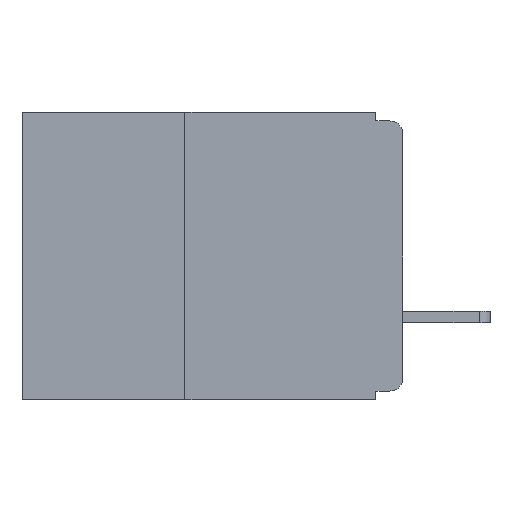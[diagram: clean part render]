
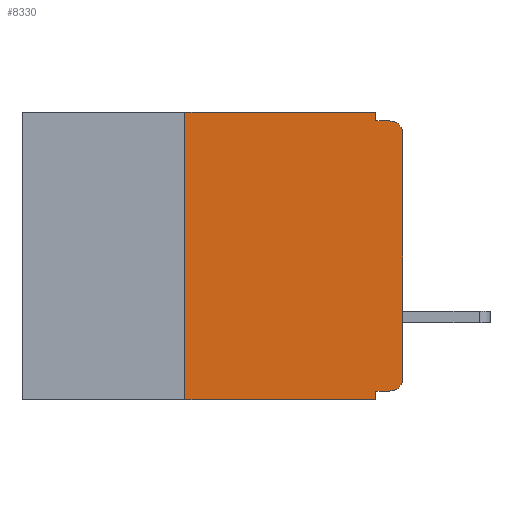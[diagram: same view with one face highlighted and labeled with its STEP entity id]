
A CAD part, left-side view. The second image highlights one B-rep face of the part: STEP entity #8330.
In plain terms, the highlighted planar face has unit normal (-1, 0, 0).
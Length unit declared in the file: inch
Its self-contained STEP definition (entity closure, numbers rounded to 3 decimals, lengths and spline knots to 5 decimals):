
#650 = LINE ( 'NONE', #17248, #4977 ) ;
#675 = ORIENTED_EDGE ( 'NONE', *, *, #1697, .T. ) ;
#850 = EDGE_CURVE ( 'NONE', #20272, #13504, #3624, .T. ) ;
#1159 = VERTEX_POINT ( 'NONE', #6246 ) ;
#1633 = AXIS2_PLACEMENT_3D ( 'NONE', #23522, #14543, #3384 ) ;
#1697 = EDGE_CURVE ( 'NONE', #17178, #10388, #9512, .T. ) ;
#1783 = LINE ( 'NONE', #21911, #15415 ) ;
#2965 = ORIENTED_EDGE ( 'NONE', *, *, #850, .F. ) ;
#3384 = DIRECTION ( 'NONE',  ( 0., 0., -1. ) ) ;
#3624 = LINE ( 'NONE', #14983, #22013 ) ;
#3762 = VERTEX_POINT ( 'NONE', #18606 ) ;
#4073 = LINE ( 'NONE', #21088, #13419 ) ;
#4673 = EDGE_CURVE ( 'NONE', #13071, #1159, #1783, .T. ) ;
#4823 = VECTOR ( 'NONE', #6919, 39.37008 ) ;
#4966 = ORIENTED_EDGE ( 'NONE', *, *, #10461, .T. ) ;
#4977 = VECTOR ( 'NONE', #9965, 39.37008 ) ;
#6220 = VECTOR ( 'NONE', #15174, 39.37008 ) ;
#6246 = CARTESIAN_POINT ( 'NONE',  ( 0., 0.25, 0. ) ) ;
#6919 = DIRECTION ( 'NONE',  ( 0., 1., 0. ) ) ;
#7081 = LINE ( 'NONE', #10183, #16347 ) ;
#7742 = FACE_OUTER_BOUND ( 'NONE', #14845, .T. ) ;
#7944 = CIRCLE ( 'NONE', #21396, 0.015 ) ;
#8330 = ADVANCED_FACE ( 'NONE', ( #7742 ), #16301, .F. ) ;
#9512 = CIRCLE ( 'NONE', #16592, 0.015 ) ;
#9738 = CARTESIAN_POINT ( 'NONE',  ( 0., 0.015, -0.025 ) ) ;
#9762 = CARTESIAN_POINT ( 'NONE',  ( 0., 0.25, -0.33 ) ) ;
#9819 = LINE ( 'NONE', #12503, #4823 ) ;
#9965 = DIRECTION ( 'NONE',  ( 0., -1., 0. ) ) ;
#10183 = CARTESIAN_POINT ( 'NONE',  ( 0., 0., -0.01 ) ) ;
#10388 = VERTEX_POINT ( 'NONE', #15047 ) ;
#10461 = EDGE_CURVE ( 'NONE', #3762, #15652, #7944, .T. ) ;
#11070 = CARTESIAN_POINT ( 'NONE',  ( 0., 0.031, 0. ) ) ;
#11258 = EDGE_CURVE ( 'NONE', #19746, #11695, #4073, .T. ) ;
#11275 = CARTESIAN_POINT ( 'NONE',  ( 0., 0.437, 0. ) ) ;
#11535 = CARTESIAN_POINT ( 'NONE',  ( 0., 0.015, -0.32 ) ) ;
#11639 = DIRECTION ( 'NONE',  ( 0., 0., -1. ) ) ;
#11695 = VERTEX_POINT ( 'NONE', #14999 ) ;
#12277 = CARTESIAN_POINT ( 'NONE',  ( 0., 0.015, -0.01 ) ) ;
#12503 = CARTESIAN_POINT ( 'NONE',  ( 0., 0., -0.32 ) ) ;
#12838 = EDGE_CURVE ( 'NONE', #1159, #19746, #16745, .T. ) ;
#12869 = ORIENTED_EDGE ( 'NONE', *, *, #11258, .F. ) ;
#13071 = VERTEX_POINT ( 'NONE', #9762 ) ;
#13159 = ORIENTED_EDGE ( 'NONE', *, *, #17260, .T. ) ;
#13350 = CARTESIAN_POINT ( 'NONE',  ( 0., 0., 0. ) ) ;
#13419 = VECTOR ( 'NONE', #22865, 39.37008 ) ;
#13504 = VERTEX_POINT ( 'NONE', #14655 ) ;
#13701 = ORIENTED_EDGE ( 'NONE', *, *, #20517, .T. ) ;
#13849 = DIRECTION ( 'NONE',  ( 0., 0., -1. ) ) ;
#14543 = DIRECTION ( 'NONE',  ( 1., 0., 0. ) ) ;
#14655 = CARTESIAN_POINT ( 'NONE',  ( 0., 0.031, -0.33 ) ) ;
#14845 = EDGE_LOOP ( 'NONE', ( #13701, #4966, #16558, #12869, #23028, #21634, #13159, #2965, #21098, #675 ) ) ;
#14864 = DIRECTION ( 'NONE',  ( 0., -1., 0. ) ) ;
#14983 = CARTESIAN_POINT ( 'NONE',  ( 0., 0.031, -0.33 ) ) ;
#14999 = CARTESIAN_POINT ( 'NONE',  ( 0., 0.031, -0.01 ) ) ;
#15047 = CARTESIAN_POINT ( 'NONE',  ( 0., 0., -0.305 ) ) ;
#15174 = DIRECTION ( 'NONE',  ( 0., 0., 1. ) ) ;
#15415 = VECTOR ( 'NONE', #20446, 39.37008 ) ;
#15652 = VERTEX_POINT ( 'NONE', #12277 ) ;
#16138 = EDGE_CURVE ( 'NONE', #11695, #15652, #7081, .T. ) ;
#16301 = PLANE ( 'NONE',  #1633 ) ;
#16347 = VECTOR ( 'NONE', #22935, 39.37008 ) ;
#16558 = ORIENTED_EDGE ( 'NONE', *, *, #16138, .F. ) ;
#16592 = AXIS2_PLACEMENT_3D ( 'NONE', #23579, #20659, #17983 ) ;
#16745 = LINE ( 'NONE', #11275, #20968 ) ;
#17178 = VERTEX_POINT ( 'NONE', #11535 ) ;
#17248 = CARTESIAN_POINT ( 'NONE',  ( 0., 0.437, -0.33 ) ) ;
#17260 = EDGE_CURVE ( 'NONE', #13071, #13504, #650, .T. ) ;
#17983 = DIRECTION ( 'NONE',  ( 0., 0., -1. ) ) ;
#18606 = CARTESIAN_POINT ( 'NONE',  ( 0., 0., -0.025 ) ) ;
#19746 = VERTEX_POINT ( 'NONE', #11070 ) ;
#20206 = EDGE_CURVE ( 'NONE', #17178, #20272, #9819, .T. ) ;
#20272 = VERTEX_POINT ( 'NONE', #21728 ) ;
#20446 = DIRECTION ( 'NONE',  ( 0., 0., 1. ) ) ;
#20517 = EDGE_CURVE ( 'NONE', #10388, #3762, #20895, .T. ) ;
#20659 = DIRECTION ( 'NONE',  ( -1., 0., 0. ) ) ;
#20895 = LINE ( 'NONE', #13350, #6220 ) ;
#20968 = VECTOR ( 'NONE', #14864, 39.37008 ) ;
#21088 = CARTESIAN_POINT ( 'NONE',  ( 0., 0.031, 0. ) ) ;
#21098 = ORIENTED_EDGE ( 'NONE', *, *, #20206, .F. ) ;
#21396 = AXIS2_PLACEMENT_3D ( 'NONE', #9738, #22441, #11639 ) ;
#21634 = ORIENTED_EDGE ( 'NONE', *, *, #4673, .F. ) ;
#21728 = CARTESIAN_POINT ( 'NONE',  ( 0., 0.031, -0.32 ) ) ;
#21911 = CARTESIAN_POINT ( 'NONE',  ( 0., 0.25, -0.33 ) ) ;
#22013 = VECTOR ( 'NONE', #13849, 39.37008 ) ;
#22441 = DIRECTION ( 'NONE',  ( -1., 0., 0. ) ) ;
#22865 = DIRECTION ( 'NONE',  ( 0., 0., -1. ) ) ;
#22935 = DIRECTION ( 'NONE',  ( 0., -1., 0. ) ) ;
#23028 = ORIENTED_EDGE ( 'NONE', *, *, #12838, .F. ) ;
#23522 = CARTESIAN_POINT ( 'NONE',  ( 0., 0.437, 0. ) ) ;
#23579 = CARTESIAN_POINT ( 'NONE',  ( 0., 0.015, -0.305 ) ) ;
